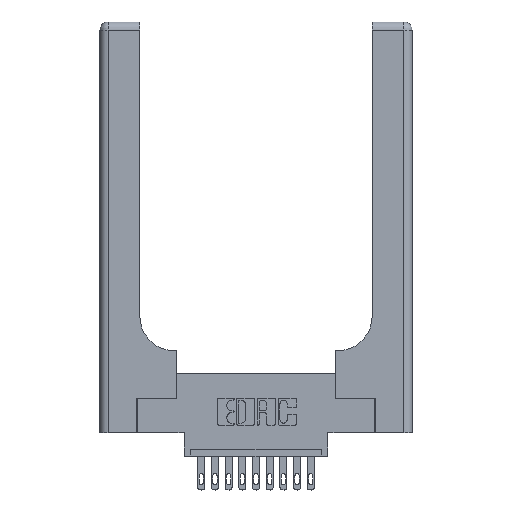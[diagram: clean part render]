
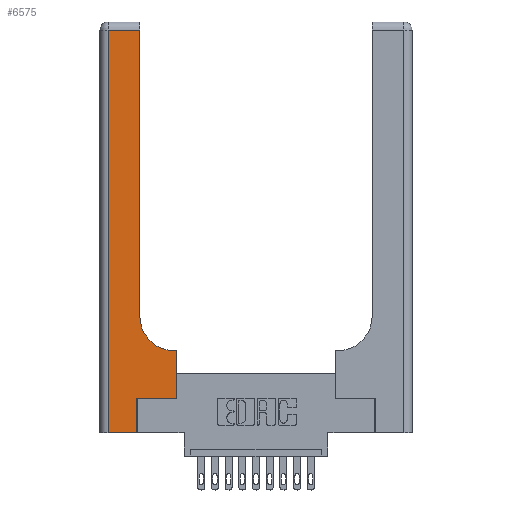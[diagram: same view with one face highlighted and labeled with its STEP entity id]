
A CAD part, top view. The second image highlights one B-rep face of the part: STEP entity #6575.
In plain terms, the highlighted planar face has unit normal (0, 0, 1).
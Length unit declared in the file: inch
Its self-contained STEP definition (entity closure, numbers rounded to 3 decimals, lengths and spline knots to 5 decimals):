
#186 = LINE ( 'NONE', #11259, #15504 ) ;
#230 = CARTESIAN_POINT ( 'NONE',  ( 0.06, 2.94, 0.37 ) ) ;
#604 = FACE_OUTER_BOUND ( 'NONE', #7718, .T. ) ;
#1129 = CARTESIAN_POINT ( 'NONE',  ( 0.2915, 2.94, 0.37 ) ) ;
#1175 = VERTEX_POINT ( 'NONE', #1129 ) ;
#1282 = VERTEX_POINT ( 'NONE', #12137 ) ;
#1289 = VECTOR ( 'NONE', #1904, 39.37008 ) ;
#1579 = EDGE_CURVE ( 'NONE', #2045, #7448, #15509, .T. ) ;
#1623 = CIRCLE ( 'NONE', #3462, 0.25 ) ;
#1739 = CARTESIAN_POINT ( 'NONE',  ( 0.06, 3., 0.37 ) ) ;
#1771 = ORIENTED_EDGE ( 'NONE', *, *, #4666, .T. ) ;
#1887 = LINE ( 'NONE', #1739, #1289 ) ;
#1904 = DIRECTION ( 'NONE',  ( 0., -1., 0. ) ) ;
#2045 = VERTEX_POINT ( 'NONE', #15552 ) ;
#2061 = ORIENTED_EDGE ( 'NONE', *, *, #14996, .T. ) ;
#2075 = CARTESIAN_POINT ( 'NONE',  ( 0., 3., 0.37 ) ) ;
#2734 = VECTOR ( 'NONE', #10209, 39.37008 ) ;
#2757 = VERTEX_POINT ( 'NONE', #10195 ) ;
#3338 = VECTOR ( 'NONE', #15208, 39.37008 ) ;
#3341 = DIRECTION ( 'NONE',  ( 0., 1., 0. ) ) ;
#3348 = EDGE_CURVE ( 'NONE', #4878, #12178, #7534, .T. ) ;
#3462 = AXIS2_PLACEMENT_3D ( 'NONE', #3979, #8883, #12799 ) ;
#3511 = PLANE ( 'NONE',  #8992 ) ;
#3906 = DIRECTION ( 'NONE',  ( -1., 0., 0. ) ) ;
#3979 = CARTESIAN_POINT ( 'NONE',  ( 0.5415, 0.85, 0.37 ) ) ;
#4229 = ORIENTED_EDGE ( 'NONE', *, *, #3348, .T. ) ;
#4291 = CARTESIAN_POINT ( 'NONE',  ( 0.06, 0., 0.37 ) ) ;
#4666 = EDGE_CURVE ( 'NONE', #1282, #4878, #9464, .T. ) ;
#4878 = VERTEX_POINT ( 'NONE', #11399 ) ;
#5091 = LINE ( 'NONE', #13497, #15038 ) ;
#6053 = CARTESIAN_POINT ( 'NONE',  ( 0.2915, 0.6, 0.37 ) ) ;
#6328 = ORIENTED_EDGE ( 'NONE', *, *, #1579, .T. ) ;
#6575 = ADVANCED_FACE ( 'NONE', ( #604 ), #3511, .F. ) ;
#7132 = EDGE_CURVE ( 'NONE', #7448, #2757, #1623, .T. ) ;
#7341 = VERTEX_POINT ( 'NONE', #4291 ) ;
#7448 = VERTEX_POINT ( 'NONE', #10660 ) ;
#7534 = LINE ( 'NONE', #15092, #3338 ) ;
#7718 = EDGE_LOOP ( 'NONE', ( #13376, #2061, #12620, #12270, #1771, #4229, #9155, #6328, #9042 ) ) ;
#8403 = VERTEX_POINT ( 'NONE', #230 ) ;
#8425 = CARTESIAN_POINT ( 'NONE',  ( 0.5585, 0.25, 0.37 ) ) ;
#8883 = DIRECTION ( 'NONE',  ( 0., 0., -1. ) ) ;
#8992 = AXIS2_PLACEMENT_3D ( 'NONE', #2075, #14949, #11035 ) ;
#9042 = ORIENTED_EDGE ( 'NONE', *, *, #7132, .T. ) ;
#9068 = VECTOR ( 'NONE', #13311, 39.37008 ) ;
#9155 = ORIENTED_EDGE ( 'NONE', *, *, #15362, .T. ) ;
#9387 = CARTESIAN_POINT ( 'NONE',  ( 0.269, 0., 0.37 ) ) ;
#9464 = LINE ( 'NONE', #9387, #9068 ) ;
#10195 = CARTESIAN_POINT ( 'NONE',  ( 0.2915, 0.85, 0.37 ) ) ;
#10209 = DIRECTION ( 'NONE',  ( 1., 0., 0. ) ) ;
#10257 = LINE ( 'NONE', #12734, #16234 ) ;
#10660 = CARTESIAN_POINT ( 'NONE',  ( 0.5415, 0.6, 0.37 ) ) ;
#11035 = DIRECTION ( 'NONE',  ( -1., 0., 0. ) ) ;
#11171 = EDGE_CURVE ( 'NONE', #8403, #7341, #1887, .T. ) ;
#11259 = CARTESIAN_POINT ( 'NONE',  ( 0.2915, 3., 0.37 ) ) ;
#11399 = CARTESIAN_POINT ( 'NONE',  ( 0.269, 0.25, 0.37 ) ) ;
#11647 = LINE ( 'NONE', #14382, #2734 ) ;
#11923 = EDGE_CURVE ( 'NONE', #2757, #1175, #186, .T. ) ;
#12114 = VECTOR ( 'NONE', #13540, 39.37008 ) ;
#12137 = CARTESIAN_POINT ( 'NONE',  ( 0.269, 0., 0.37 ) ) ;
#12178 = VERTEX_POINT ( 'NONE', #8425 ) ;
#12270 = ORIENTED_EDGE ( 'NONE', *, *, #14042, .T. ) ;
#12620 = ORIENTED_EDGE ( 'NONE', *, *, #11171, .T. ) ;
#12734 = CARTESIAN_POINT ( 'NONE',  ( 0., 2.94, 0.37 ) ) ;
#12799 = DIRECTION ( 'NONE',  ( 1., 0., 0. ) ) ;
#13311 = DIRECTION ( 'NONE',  ( 0., 1., 0. ) ) ;
#13376 = ORIENTED_EDGE ( 'NONE', *, *, #11923, .T. ) ;
#13497 = CARTESIAN_POINT ( 'NONE',  ( 0.5585, 0.25, 0.37 ) ) ;
#13540 = DIRECTION ( 'NONE',  ( -1., 0., 0. ) ) ;
#14042 = EDGE_CURVE ( 'NONE', #7341, #1282, #11647, .T. ) ;
#14045 = DIRECTION ( 'NONE',  ( 0., 1., 0. ) ) ;
#14382 = CARTESIAN_POINT ( 'NONE',  ( 0., 0., 0.37 ) ) ;
#14949 = DIRECTION ( 'NONE',  ( 0., 0., -1. ) ) ;
#14996 = EDGE_CURVE ( 'NONE', #1175, #8403, #10257, .T. ) ;
#15038 = VECTOR ( 'NONE', #3341, 39.37008 ) ;
#15092 = CARTESIAN_POINT ( 'NONE',  ( 0.269, 0.25, 0.37 ) ) ;
#15208 = DIRECTION ( 'NONE',  ( 1., 0., 0. ) ) ;
#15362 = EDGE_CURVE ( 'NONE', #12178, #2045, #5091, .T. ) ;
#15504 = VECTOR ( 'NONE', #14045, 39.37008 ) ;
#15509 = LINE ( 'NONE', #6053, #12114 ) ;
#15552 = CARTESIAN_POINT ( 'NONE',  ( 0.5585, 0.6, 0.37 ) ) ;
#16234 = VECTOR ( 'NONE', #3906, 39.37008 ) ;
